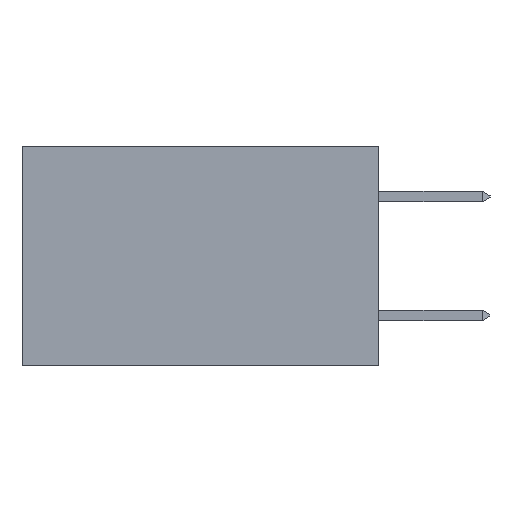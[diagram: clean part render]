
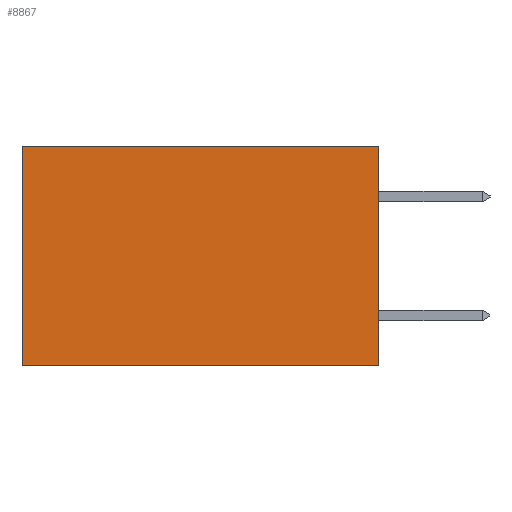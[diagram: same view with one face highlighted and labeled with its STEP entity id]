
A CAD part, left-side view. The second image highlights one B-rep face of the part: STEP entity #8867.
In plain terms, the highlighted planar face has unit normal (-1, 0, 0).
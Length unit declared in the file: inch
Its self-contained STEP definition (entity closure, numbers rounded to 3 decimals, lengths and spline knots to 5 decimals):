
#493 = VECTOR ( 'NONE', #9993, 39.37008 ) ;
#514 = VECTOR ( 'NONE', #22768, 39.37008 ) ;
#961 = CARTESIAN_POINT ( 'NONE',  ( 0.298, 0., 0. ) ) ;
#1139 = DIRECTION ( 'NONE',  ( 1., 0., 0. ) ) ;
#3167 = CARTESIAN_POINT ( 'NONE',  ( 0.298, 0., 0. ) ) ;
#3838 = VECTOR ( 'NONE', #19785, 39.37008 ) ;
#5603 = VERTEX_POINT ( 'NONE', #7886 ) ;
#5878 = EDGE_CURVE ( 'NONE', #10432, #16699, #18160, .T. ) ;
#6091 = DIRECTION ( 'NONE',  ( 0., 0., -1. ) ) ;
#6146 = VECTOR ( 'NONE', #10132, 39.37008 ) ;
#6258 = EDGE_CURVE ( 'NONE', #5603, #10432, #10226, .T. ) ;
#7368 = PLANE ( 'NONE',  #26929 ) ;
#7703 = CARTESIAN_POINT ( 'NONE',  ( 0.298, 0.6, 0. ) ) ;
#7886 = CARTESIAN_POINT ( 'NONE',  ( 0.298, 0., 0. ) ) ;
#8461 = CARTESIAN_POINT ( 'NONE',  ( 0.298, 0., 0. ) ) ;
#8512 = VERTEX_POINT ( 'NONE', #25375 ) ;
#8867 = ADVANCED_FACE ( 'NONE', ( #29861 ), #7368, .F. ) ;
#9005 = CARTESIAN_POINT ( 'NONE',  ( 0.298, 0., -0.37 ) ) ;
#9993 = DIRECTION ( 'NONE',  ( 0., 1., 0. ) ) ;
#10132 = DIRECTION ( 'NONE',  ( 0., 0., -1. ) ) ;
#10226 = LINE ( 'NONE', #961, #3838 ) ;
#10432 = VERTEX_POINT ( 'NONE', #9005 ) ;
#11205 = EDGE_CURVE ( 'NONE', #8512, #16699, #12510, .T. ) ;
#12510 = LINE ( 'NONE', #7703, #6146 ) ;
#12640 = LINE ( 'NONE', #8461, #514 ) ;
#12676 = EDGE_CURVE ( 'NONE', #5603, #8512, #12640, .T. ) ;
#14273 = EDGE_LOOP ( 'NONE', ( #19229, #20391, #23522, #20899 ) ) ;
#14771 = CARTESIAN_POINT ( 'NONE',  ( 0.298, 0., -0.37 ) ) ;
#16699 = VERTEX_POINT ( 'NONE', #27298 ) ;
#18160 = LINE ( 'NONE', #14771, #493 ) ;
#19229 = ORIENTED_EDGE ( 'NONE', *, *, #11205, .T. ) ;
#19785 = DIRECTION ( 'NONE',  ( 0., 0., -1. ) ) ;
#20391 = ORIENTED_EDGE ( 'NONE', *, *, #5878, .F. ) ;
#20899 = ORIENTED_EDGE ( 'NONE', *, *, #12676, .T. ) ;
#22768 = DIRECTION ( 'NONE',  ( 0., 1., 0. ) ) ;
#23522 = ORIENTED_EDGE ( 'NONE', *, *, #6258, .F. ) ;
#25375 = CARTESIAN_POINT ( 'NONE',  ( 0.298, 0.6, 0. ) ) ;
#26929 = AXIS2_PLACEMENT_3D ( 'NONE', #3167, #1139, #6091 ) ;
#27298 = CARTESIAN_POINT ( 'NONE',  ( 0.298, 0.6, -0.37 ) ) ;
#29861 = FACE_OUTER_BOUND ( 'NONE', #14273, .T. ) ;
